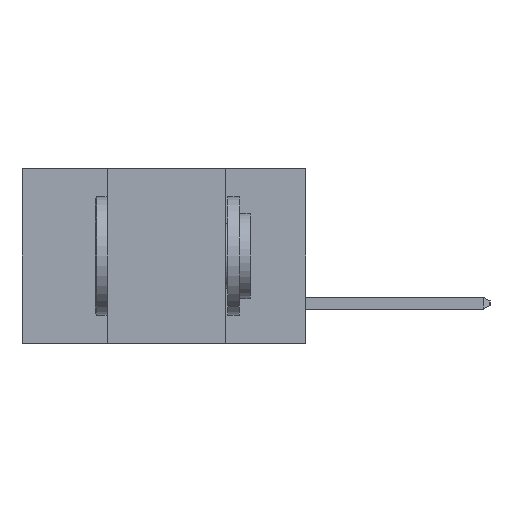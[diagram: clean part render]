
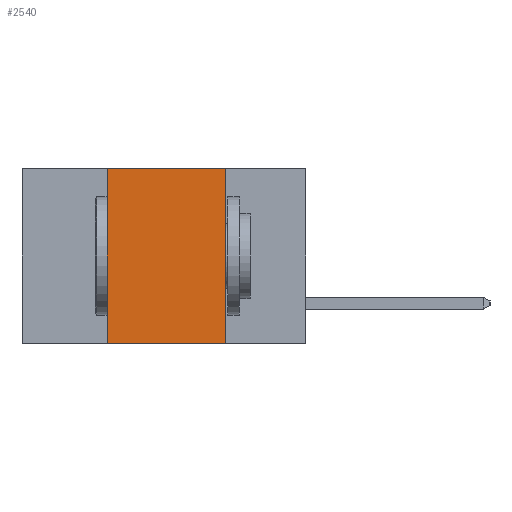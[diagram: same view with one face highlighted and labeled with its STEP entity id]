
A CAD part, left-side view. The second image highlights one B-rep face of the part: STEP entity #2540.
In plain terms, the highlighted planar face has unit normal (-1, 0, 0).
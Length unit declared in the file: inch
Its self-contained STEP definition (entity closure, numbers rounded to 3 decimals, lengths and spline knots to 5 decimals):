
#226 = LINE ( 'NONE', #2851, #10076 ) ;
#284 = VERTEX_POINT ( 'NONE', #7227 ) ;
#425 = VERTEX_POINT ( 'NONE', #5178 ) ;
#513 = CARTESIAN_POINT ( 'NONE',  ( 0., 0.42, -0.37 ) ) ;
#625 = DIRECTION ( 'NONE',  ( 0., -1., 0. ) ) ;
#946 = CARTESIAN_POINT ( 'NONE',  ( 0., 0.6, 0. ) ) ;
#1795 = VERTEX_POINT ( 'NONE', #5598 ) ;
#2029 = VERTEX_POINT ( 'NONE', #5482 ) ;
#2031 = ORIENTED_EDGE ( 'NONE', *, *, #5503, .F. ) ;
#2392 = PLANE ( 'NONE',  #7413 ) ;
#2540 = ADVANCED_FACE ( 'NONE', ( #13162 ), #2392, .F. ) ;
#2774 = EDGE_CURVE ( 'NONE', #425, #284, #226, .T. ) ;
#2851 = CARTESIAN_POINT ( 'NONE',  ( 0., 0.6, -0.37 ) ) ;
#4081 = LINE ( 'NONE', #513, #14973 ) ;
#4119 = DIRECTION ( 'NONE',  ( 0., 0., -1. ) ) ;
#4225 = CARTESIAN_POINT ( 'NONE',  ( 0., 0.17, -0.37 ) ) ;
#5178 = CARTESIAN_POINT ( 'NONE',  ( 0., 0.42, -0.37 ) ) ;
#5237 = EDGE_CURVE ( 'NONE', #425, #2029, #4081, .T. ) ;
#5482 = CARTESIAN_POINT ( 'NONE',  ( 0., 0.42, 0. ) ) ;
#5503 = EDGE_CURVE ( 'NONE', #2029, #1795, #10008, .T. ) ;
#5598 = CARTESIAN_POINT ( 'NONE',  ( 0., 0.17, 0. ) ) ;
#5625 = DIRECTION ( 'NONE',  ( 0., -1., 0. ) ) ;
#5898 = ORIENTED_EDGE ( 'NONE', *, *, #2774, .T. ) ;
#5965 = EDGE_CURVE ( 'NONE', #1795, #284, #6362, .T. ) ;
#5975 = VECTOR ( 'NONE', #4119, 39.37008 ) ;
#6362 = LINE ( 'NONE', #4225, #5975 ) ;
#7227 = CARTESIAN_POINT ( 'NONE',  ( 0., 0.17, -0.37 ) ) ;
#7413 = AXIS2_PLACEMENT_3D ( 'NONE', #14616, #13581, #12624 ) ;
#10008 = LINE ( 'NONE', #946, #13270 ) ;
#10076 = VECTOR ( 'NONE', #5625, 39.37008 ) ;
#11067 = ORIENTED_EDGE ( 'NONE', *, *, #5965, .F. ) ;
#11084 = EDGE_LOOP ( 'NONE', ( #11067, #2031, #15789, #5898 ) ) ;
#12624 = DIRECTION ( 'NONE',  ( 0., 0., -1. ) ) ;
#13162 = FACE_OUTER_BOUND ( 'NONE', #11084, .T. ) ;
#13270 = VECTOR ( 'NONE', #625, 39.37008 ) ;
#13581 = DIRECTION ( 'NONE',  ( 1., 0., 0. ) ) ;
#14387 = DIRECTION ( 'NONE',  ( 0., 0., 1. ) ) ;
#14616 = CARTESIAN_POINT ( 'NONE',  ( 0., 0.6, 0. ) ) ;
#14973 = VECTOR ( 'NONE', #14387, 39.37008 ) ;
#15789 = ORIENTED_EDGE ( 'NONE', *, *, #5237, .F. ) ;
